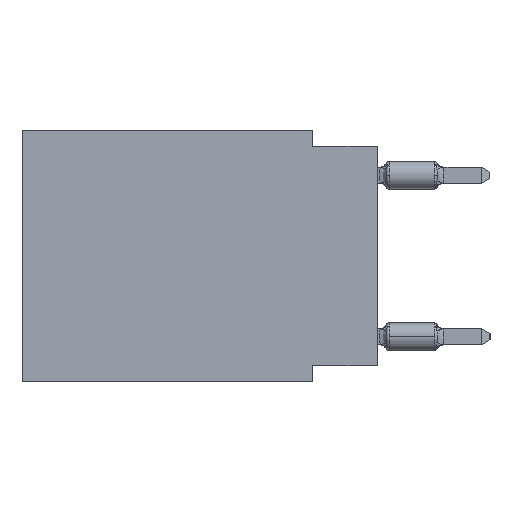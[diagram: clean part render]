
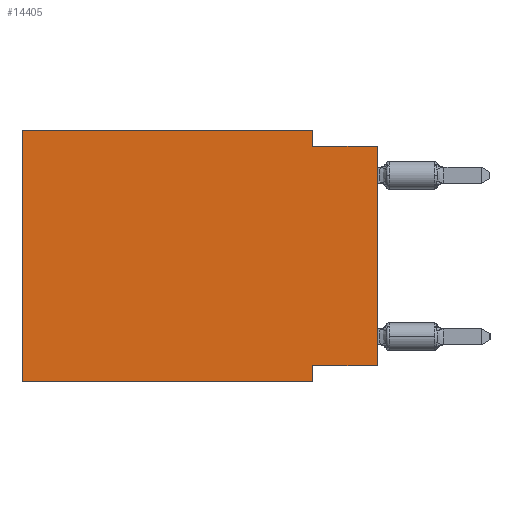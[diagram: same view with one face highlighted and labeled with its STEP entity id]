
A CAD part, left-side view. The second image highlights one B-rep face of the part: STEP entity #14405.
In plain terms, the highlighted planar face has unit normal (-1, 0, 0).
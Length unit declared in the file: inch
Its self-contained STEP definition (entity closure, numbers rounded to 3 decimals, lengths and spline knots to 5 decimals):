
#300 = DIRECTION ( 'NONE',  ( 0., -1., 0. ) ) ;
#1324 = CARTESIAN_POINT ( 'NONE',  ( 0., 0., -0.025 ) ) ;
#1399 = VERTEX_POINT ( 'NONE', #11509 ) ;
#3301 = VECTOR ( 'NONE', #300, 39.37008 ) ;
#3528 = EDGE_LOOP ( 'NONE', ( #11155, #4819, #31042, #8795, #13191, #12831, #23578, #22150 ) ) ;
#3690 = CARTESIAN_POINT ( 'NONE',  ( 0., 0.1, -0.025 ) ) ;
#3823 = AXIS2_PLACEMENT_3D ( 'NONE', #18018, #17699, #5179 ) ;
#4182 = LINE ( 'NONE', #23996, #15944 ) ;
#4740 = LINE ( 'NONE', #1324, #9640 ) ;
#4819 = ORIENTED_EDGE ( 'NONE', *, *, #16302, .F. ) ;
#5070 = CARTESIAN_POINT ( 'NONE',  ( 0., 0., -0.365 ) ) ;
#5179 = DIRECTION ( 'NONE',  ( 0., 0., -1. ) ) ;
#5769 = CARTESIAN_POINT ( 'NONE',  ( 0., 0., -0.025 ) ) ;
#5906 = EDGE_CURVE ( 'NONE', #16547, #1399, #6327, .T. ) ;
#6327 = LINE ( 'NONE', #11414, #29073 ) ;
#6910 = CARTESIAN_POINT ( 'NONE',  ( 0., 0., -0.365 ) ) ;
#7456 = LINE ( 'NONE', #12885, #3301 ) ;
#7487 = LINE ( 'NONE', #17509, #31975 ) ;
#7867 = VERTEX_POINT ( 'NONE', #30923 ) ;
#8552 = CARTESIAN_POINT ( 'NONE',  ( 0., 0., 0. ) ) ;
#8795 = ORIENTED_EDGE ( 'NONE', *, *, #30530, .F. ) ;
#9640 = VECTOR ( 'NONE', #29446, 39.37008 ) ;
#11155 = ORIENTED_EDGE ( 'NONE', *, *, #22601, .T. ) ;
#11414 = CARTESIAN_POINT ( 'NONE',  ( 0., 0.55, -0.39 ) ) ;
#11509 = CARTESIAN_POINT ( 'NONE',  ( 0., 0.1, -0.39 ) ) ;
#11895 = VERTEX_POINT ( 'NONE', #23891 ) ;
#12831 = ORIENTED_EDGE ( 'NONE', *, *, #5906, .T. ) ;
#12832 = DIRECTION ( 'NONE',  ( 0., 1., 0. ) ) ;
#12885 = CARTESIAN_POINT ( 'NONE',  ( 0., 0.55, 0. ) ) ;
#13191 = ORIENTED_EDGE ( 'NONE', *, *, #28789, .F. ) ;
#14405 = ADVANCED_FACE ( 'NONE', ( #22664 ), #20189, .F. ) ;
#14764 = LINE ( 'NONE', #14928, #26190 ) ;
#14928 = CARTESIAN_POINT ( 'NONE',  ( 0., 0.1, -0.39 ) ) ;
#15944 = VECTOR ( 'NONE', #18999, 39.37008 ) ;
#16302 = EDGE_CURVE ( 'NONE', #28679, #16543, #4740, .T. ) ;
#16334 = VERTEX_POINT ( 'NONE', #6910 ) ;
#16543 = VERTEX_POINT ( 'NONE', #5769 ) ;
#16547 = VERTEX_POINT ( 'NONE', #22329 ) ;
#17509 = CARTESIAN_POINT ( 'NONE',  ( 0., 0.1, 0. ) ) ;
#17699 = DIRECTION ( 'NONE',  ( 1., 0., 0. ) ) ;
#18018 = CARTESIAN_POINT ( 'NONE',  ( 0., 0.55, 0. ) ) ;
#18559 = EDGE_CURVE ( 'NONE', #20883, #1399, #14764, .T. ) ;
#18999 = DIRECTION ( 'NONE',  ( 0., 0., 1. ) ) ;
#19065 = VECTOR ( 'NONE', #12832, 39.37008 ) ;
#20189 = PLANE ( 'NONE',  #3823 ) ;
#20883 = VERTEX_POINT ( 'NONE', #20940 ) ;
#20940 = CARTESIAN_POINT ( 'NONE',  ( 0., 0.1, -0.365 ) ) ;
#21069 = LINE ( 'NONE', #8552, #22597 ) ;
#21459 = EDGE_CURVE ( 'NONE', #11895, #28679, #7487, .T. ) ;
#22150 = ORIENTED_EDGE ( 'NONE', *, *, #28083, .F. ) ;
#22329 = CARTESIAN_POINT ( 'NONE',  ( 0., 0.55, -0.39 ) ) ;
#22597 = VECTOR ( 'NONE', #28612, 39.37008 ) ;
#22601 = EDGE_CURVE ( 'NONE', #16334, #16543, #21069, .T. ) ;
#22664 = FACE_OUTER_BOUND ( 'NONE', #3528, .T. ) ;
#23039 = LINE ( 'NONE', #5070, #19065 ) ;
#23578 = ORIENTED_EDGE ( 'NONE', *, *, #18559, .F. ) ;
#23891 = CARTESIAN_POINT ( 'NONE',  ( 0., 0.1, 0. ) ) ;
#23996 = CARTESIAN_POINT ( 'NONE',  ( 0., 0.55, 0. ) ) ;
#24993 = DIRECTION ( 'NONE',  ( 0., 0., -1. ) ) ;
#26190 = VECTOR ( 'NONE', #24993, 39.37008 ) ;
#28083 = EDGE_CURVE ( 'NONE', #16334, #20883, #23039, .T. ) ;
#28612 = DIRECTION ( 'NONE',  ( 0., 0., 1. ) ) ;
#28679 = VERTEX_POINT ( 'NONE', #3690 ) ;
#28789 = EDGE_CURVE ( 'NONE', #16547, #7867, #4182, .T. ) ;
#29073 = VECTOR ( 'NONE', #31471, 39.37008 ) ;
#29446 = DIRECTION ( 'NONE',  ( 0., -1., 0. ) ) ;
#29861 = DIRECTION ( 'NONE',  ( 0., 0., -1. ) ) ;
#30530 = EDGE_CURVE ( 'NONE', #7867, #11895, #7456, .T. ) ;
#30923 = CARTESIAN_POINT ( 'NONE',  ( 0., 0.55, 0. ) ) ;
#31042 = ORIENTED_EDGE ( 'NONE', *, *, #21459, .F. ) ;
#31471 = DIRECTION ( 'NONE',  ( 0., -1., 0. ) ) ;
#31975 = VECTOR ( 'NONE', #29861, 39.37008 ) ;
